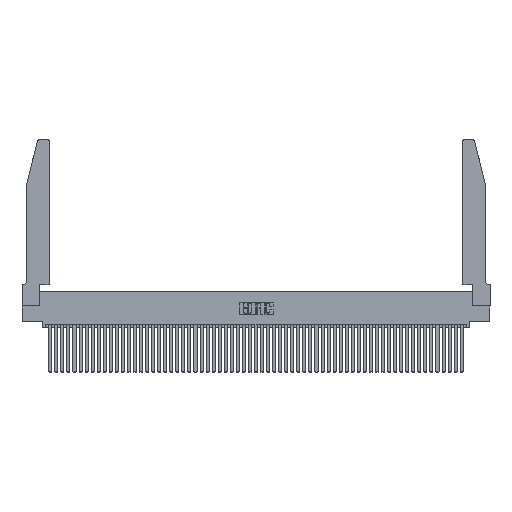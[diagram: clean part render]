
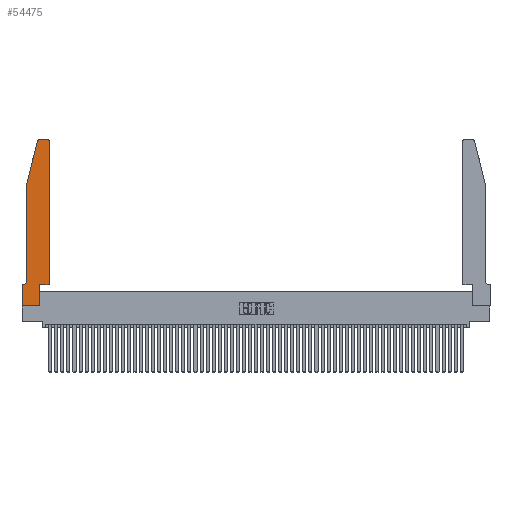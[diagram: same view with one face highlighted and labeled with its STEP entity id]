
A CAD part, top view. The second image highlights one B-rep face of the part: STEP entity #54475.
In plain terms, the highlighted planar face has unit normal (0, 0, 1).
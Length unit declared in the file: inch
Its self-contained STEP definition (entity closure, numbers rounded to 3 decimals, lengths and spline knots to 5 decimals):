
#533 = PLANE ( 'NONE',  #9118 ) ;
#661 = EDGE_CURVE ( 'NONE', #10391, #34980, #48845, .T. ) ;
#685 = VECTOR ( 'NONE', #29205, 39.37008 ) ;
#713 = DIRECTION ( 'NONE',  ( 0., 0., 1. ) ) ;
#1471 = LINE ( 'NONE', #32583, #22226 ) ;
#1887 = EDGE_CURVE ( 'NONE', #34980, #30226, #52698, .T. ) ;
#3332 = CARTESIAN_POINT ( 'NONE',  ( 0.284, 2.72, 0.37 ) ) ;
#3457 = LINE ( 'NONE', #37251, #32753 ) ;
#3585 = VERTEX_POINT ( 'NONE', #45647 ) ;
#3780 = EDGE_CURVE ( 'NONE', #53961, #27368, #7112, .T. ) ;
#4102 = VERTEX_POINT ( 'NONE', #45386 ) ;
#5269 = EDGE_CURVE ( 'NONE', #7837, #19327, #44388, .T. ) ;
#5365 = CARTESIAN_POINT ( 'NONE',  ( 0.4205, 2.72, 0.37 ) ) ;
#5943 = ORIENTED_EDGE ( 'NONE', *, *, #34712, .T. ) ;
#5986 = ORIENTED_EDGE ( 'NONE', *, *, #40642, .T. ) ;
#6293 = VERTEX_POINT ( 'NONE', #34535 ) ;
#6936 = ORIENTED_EDGE ( 'NONE', *, *, #26007, .T. ) ;
#7112 = LINE ( 'NONE', #26437, #34112 ) ;
#7267 = LINE ( 'NONE', #15055, #51288 ) ;
#7501 = DIRECTION ( 'NONE',  ( 0., 0., -1. ) ) ;
#7518 = ORIENTED_EDGE ( 'NONE', *, *, #54980, .T. ) ;
#7837 = VERTEX_POINT ( 'NONE', #22697 ) ;
#8023 = CARTESIAN_POINT ( 'NONE',  ( 0., 0., 0.37 ) ) ;
#9118 = AXIS2_PLACEMENT_3D ( 'NONE', #48075, #713, #9520 ) ;
#9463 = VERTEX_POINT ( 'NONE', #23701 ) ;
#9520 = DIRECTION ( 'NONE',  ( 1., 0., 0. ) ) ;
#10391 = VERTEX_POINT ( 'NONE', #37549 ) ;
#11873 = CARTESIAN_POINT ( 'NONE',  ( 0.4505, 0.35, 0.37 ) ) ;
#12044 = EDGE_LOOP ( 'NONE', ( #50637, #36514, #41330, #23692, #6936, #5943, #7518, #32252, #16389, #12763, #31513, #5986 ) ) ;
#12071 = CIRCLE ( 'NONE', #28288, 0.07 ) ;
#12763 = ORIENTED_EDGE ( 'NONE', *, *, #50079, .T. ) ;
#14518 = AXIS2_PLACEMENT_3D ( 'NONE', #3332, #49964, #15880 ) ;
#15055 = CARTESIAN_POINT ( 'NONE',  ( 0.0755, 0.35, 0.37 ) ) ;
#15880 = DIRECTION ( 'NONE',  ( 1., 0., 0. ) ) ;
#16253 = DIRECTION ( 'NONE',  ( -0.239, -0.971, 0. ) ) ;
#16389 = ORIENTED_EDGE ( 'NONE', *, *, #1887, .T. ) ;
#16453 = DIRECTION ( 'NONE',  ( 0., -1., 0. ) ) ;
#18399 = CARTESIAN_POINT ( 'NONE',  ( 0.25487, 2.72718, 0.37 ) ) ;
#19327 = VERTEX_POINT ( 'NONE', #18399 ) ;
#19734 = DIRECTION ( 'NONE',  ( -1., 0., 0. ) ) ;
#20176 = FACE_OUTER_BOUND ( 'NONE', #12044, .T. ) ;
#20310 = CARTESIAN_POINT ( 'NONE',  ( 0.2865, 0.35, 0.37 ) ) ;
#20596 = DIRECTION ( 'NONE',  ( -1., 0., 0. ) ) ;
#21565 = CARTESIAN_POINT ( 'NONE',  ( 0.2865, 0., 0.37 ) ) ;
#22226 = VECTOR ( 'NONE', #16253, 39.37008 ) ;
#22697 = CARTESIAN_POINT ( 'NONE',  ( 0.284, 2.75, 0.37 ) ) ;
#23356 = CARTESIAN_POINT ( 'NONE',  ( 0., 0.35, 0.37 ) ) ;
#23692 = ORIENTED_EDGE ( 'NONE', *, *, #33262, .T. ) ;
#23701 = CARTESIAN_POINT ( 'NONE',  ( 0.0055, 0.35, 0.37 ) ) ;
#24726 = EDGE_CURVE ( 'NONE', #19327, #4102, #1471, .T. ) ;
#25419 = CARTESIAN_POINT ( 'NONE',  ( 0.0055, 0.42, 0.37 ) ) ;
#26007 = EDGE_CURVE ( 'NONE', #6293, #9463, #12071, .T. ) ;
#26437 = CARTESIAN_POINT ( 'NONE',  ( 0.4505, 0.35, 0.37 ) ) ;
#27368 = VERTEX_POINT ( 'NONE', #32694 ) ;
#28288 = AXIS2_PLACEMENT_3D ( 'NONE', #25419, #7501, #20596 ) ;
#29205 = DIRECTION ( 'NONE',  ( 0., -1., 0. ) ) ;
#30012 = VECTOR ( 'NONE', #32651, 39.37008 ) ;
#30226 = VERTEX_POINT ( 'NONE', #20310 ) ;
#31338 = CARTESIAN_POINT ( 'NONE',  ( 0.4505, 0.35, 0.37 ) ) ;
#31513 = ORIENTED_EDGE ( 'NONE', *, *, #3780, .T. ) ;
#32252 = ORIENTED_EDGE ( 'NONE', *, *, #661, .T. ) ;
#32583 = CARTESIAN_POINT ( 'NONE',  ( 0.0755, 2., 0.37 ) ) ;
#32651 = DIRECTION ( 'NONE',  ( 0., 1., 0. ) ) ;
#32694 = CARTESIAN_POINT ( 'NONE',  ( 0.4505, 2.72, 0.37 ) ) ;
#32753 = VECTOR ( 'NONE', #16453, 39.37008 ) ;
#33262 = EDGE_CURVE ( 'NONE', #4102, #6293, #3457, .T. ) ;
#33870 = LINE ( 'NONE', #11873, #52571 ) ;
#34112 = VECTOR ( 'NONE', #52126, 39.37008 ) ;
#34535 = CARTESIAN_POINT ( 'NONE',  ( 0.0755, 0.42, 0.37 ) ) ;
#34712 = EDGE_CURVE ( 'NONE', #9463, #54133, #7267, .T. ) ;
#34980 = VERTEX_POINT ( 'NONE', #21565 ) ;
#35876 = DIRECTION ( 'NONE',  ( 0., 0., 1. ) ) ;
#36514 = ORIENTED_EDGE ( 'NONE', *, *, #5269, .T. ) ;
#37127 = LINE ( 'NONE', #50462, #49843 ) ;
#37251 = CARTESIAN_POINT ( 'NONE',  ( 0.0755, 2., 0.37 ) ) ;
#37549 = CARTESIAN_POINT ( 'NONE',  ( 0., 0., 0.37 ) ) ;
#37847 = CIRCLE ( 'NONE', #41498, 0.03 ) ;
#38364 = DIRECTION ( 'NONE',  ( 1., 0., 0. ) ) ;
#40642 = EDGE_CURVE ( 'NONE', #27368, #3585, #37847, .T. ) ;
#41330 = ORIENTED_EDGE ( 'NONE', *, *, #24726, .T. ) ;
#41498 = AXIS2_PLACEMENT_3D ( 'NONE', #5365, #35876, #48237 ) ;
#41872 = DIRECTION ( 'NONE',  ( -1., 0., 0. ) ) ;
#43397 = LINE ( 'NONE', #54390, #685 ) ;
#44388 = CIRCLE ( 'NONE', #14518, 0.03 ) ;
#45386 = CARTESIAN_POINT ( 'NONE',  ( 0.0755, 2., 0.37 ) ) ;
#45647 = CARTESIAN_POINT ( 'NONE',  ( 0.4205, 2.75, 0.37 ) ) ;
#45737 = EDGE_CURVE ( 'NONE', #3585, #7837, #37127, .T. ) ;
#48075 = CARTESIAN_POINT ( 'NONE',  ( 0., 0.35, 0.37 ) ) ;
#48237 = DIRECTION ( 'NONE',  ( 1., 0., 0. ) ) ;
#48845 = LINE ( 'NONE', #8023, #54856 ) ;
#49843 = VECTOR ( 'NONE', #41872, 39.37008 ) ;
#49891 = DIRECTION ( 'NONE',  ( 1., 0., 0. ) ) ;
#49964 = DIRECTION ( 'NONE',  ( 0., 0., 1. ) ) ;
#50079 = EDGE_CURVE ( 'NONE', #30226, #53961, #33870, .T. ) ;
#50462 = CARTESIAN_POINT ( 'NONE',  ( 0.2605, 2.75, 0.37 ) ) ;
#50637 = ORIENTED_EDGE ( 'NONE', *, *, #45737, .T. ) ;
#51288 = VECTOR ( 'NONE', #19734, 39.37008 ) ;
#52126 = DIRECTION ( 'NONE',  ( 0., 1., 0. ) ) ;
#52571 = VECTOR ( 'NONE', #49891, 39.37008 ) ;
#52698 = LINE ( 'NONE', #53736, #30012 ) ;
#53736 = CARTESIAN_POINT ( 'NONE',  ( 0.2865, 0.35, 0.37 ) ) ;
#53961 = VERTEX_POINT ( 'NONE', #31338 ) ;
#54133 = VERTEX_POINT ( 'NONE', #23356 ) ;
#54390 = CARTESIAN_POINT ( 'NONE',  ( 0., 0., 0.37 ) ) ;
#54475 = ADVANCED_FACE ( 'NONE', ( #20176 ), #533, .T. ) ;
#54856 = VECTOR ( 'NONE', #38364, 39.37008 ) ;
#54980 = EDGE_CURVE ( 'NONE', #54133, #10391, #43397, .T. ) ;
